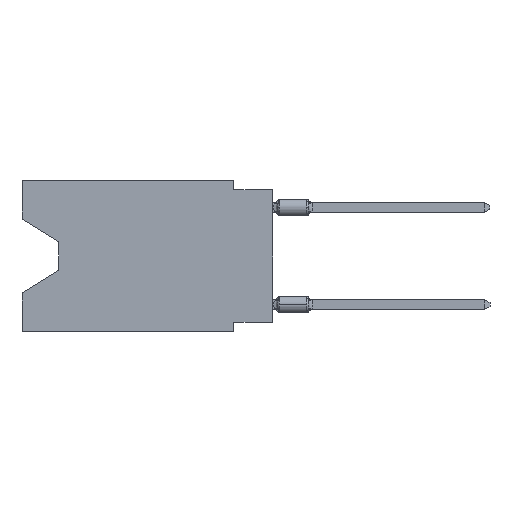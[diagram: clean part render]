
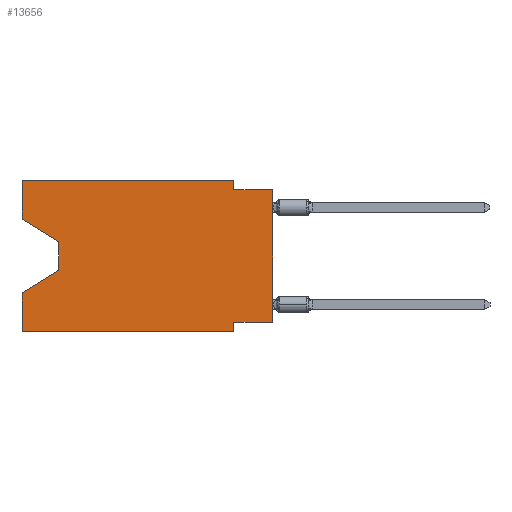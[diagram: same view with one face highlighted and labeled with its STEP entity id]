
A CAD part, left-side view. The second image highlights one B-rep face of the part: STEP entity #13656.
In plain terms, the highlighted planar face has unit normal (-1, 0, 0).
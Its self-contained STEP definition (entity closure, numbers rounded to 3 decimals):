
#213 = ORIENTED_EDGE ( 'NONE', *, *, #5521, .F. ) ;
#245 = PLANE ( 'NONE',  #2323 ) ;
#471 = LINE ( 'NONE', #8874, #9434 ) ;
#773 = LINE ( 'NONE', #6853, #8506 ) ;
#852 = DIRECTION ( 'NONE',  ( 0., 0.855, -0.519 ) ) ;
#1445 = VECTOR ( 'NONE', #23625, 1000. ) ;
#1510 = CARTESIAN_POINT ( 'NONE',  ( 0., 2.54, -9.906 ) ) ;
#1576 = CARTESIAN_POINT ( 'NONE',  ( 0., 16.383, -9.906 ) ) ;
#1768 = VECTOR ( 'NONE', #10287, 1000. ) ;
#1894 = ORIENTED_EDGE ( 'NONE', *, *, #12144, .F. ) ;
#1935 = ORIENTED_EDGE ( 'NONE', *, *, #8682, .F. ) ;
#1942 = VERTEX_POINT ( 'NONE', #14282 ) ;
#2323 = AXIS2_PLACEMENT_3D ( 'NONE', #23808, #4020, #10089 ) ;
#2403 = LINE ( 'NONE', #18314, #1768 ) ;
#2488 = CARTESIAN_POINT ( 'NONE',  ( 0., 16.383, 0. ) ) ;
#2506 = LINE ( 'NONE', #6135, #14990 ) ;
#2521 = EDGE_CURVE ( 'NONE', #8930, #2765, #773, .T. ) ;
#2765 = VERTEX_POINT ( 'NONE', #9418 ) ;
#2784 = ORIENTED_EDGE ( 'NONE', *, *, #15874, .T. ) ;
#3424 = CARTESIAN_POINT ( 'NONE',  ( 0., 2.54, 0. ) ) ;
#4020 = DIRECTION ( 'NONE',  ( 1., 0., 0. ) ) ;
#4273 = EDGE_CURVE ( 'NONE', #7052, #2765, #4348, .T. ) ;
#4348 = LINE ( 'NONE', #24664, #4438 ) ;
#4438 = VECTOR ( 'NONE', #852, 1000. ) ;
#4528 = DIRECTION ( 'NONE',  ( 0., 0., 1. ) ) ;
#5235 = LINE ( 'NONE', #3424, #25287 ) ;
#5400 = VECTOR ( 'NONE', #9411, 1000. ) ;
#5521 = EDGE_CURVE ( 'NONE', #1942, #22151, #471, .T. ) ;
#6133 = VERTEX_POINT ( 'NONE', #22689 ) ;
#6135 = CARTESIAN_POINT ( 'NONE',  ( 0., 0., -0.635 ) ) ;
#6368 = DIRECTION ( 'NONE',  ( 0., -1., 0. ) ) ;
#6853 = CARTESIAN_POINT ( 'NONE',  ( 0., 16.383, 0. ) ) ;
#7016 = EDGE_CURVE ( 'NONE', #22151, #11858, #15379, .T. ) ;
#7052 = VERTEX_POINT ( 'NONE', #24275 ) ;
#7441 = ORIENTED_EDGE ( 'NONE', *, *, #11466, .T. ) ;
#7478 = CARTESIAN_POINT ( 'NONE',  ( 0., 2.54, 0. ) ) ;
#7889 = VECTOR ( 'NONE', #24827, 1000. ) ;
#8082 = EDGE_LOOP ( 'NONE', ( #16362, #10156, #13849, #12026, #7441, #9031, #213, #2784, #1935, #17126, #1894, #15111 ) ) ;
#8506 = VECTOR ( 'NONE', #4528, 1000. ) ;
#8641 = CARTESIAN_POINT ( 'NONE',  ( 0., 13.97, -4.013 ) ) ;
#8682 = EDGE_CURVE ( 'NONE', #14234, #11019, #2506, .T. ) ;
#8874 = CARTESIAN_POINT ( 'NONE',  ( 0., 0., -9.271 ) ) ;
#8930 = VERTEX_POINT ( 'NONE', #1576 ) ;
#9031 = ORIENTED_EDGE ( 'NONE', *, *, #7016, .F. ) ;
#9411 = DIRECTION ( 'NONE',  ( 0., 0., -1. ) ) ;
#9418 = CARTESIAN_POINT ( 'NONE',  ( 0., 16.383, -7.36 ) ) ;
#9434 = VECTOR ( 'NONE', #16774, 1000. ) ;
#9471 = VERTEX_POINT ( 'NONE', #7478 ) ;
#10089 = DIRECTION ( 'NONE',  ( 0., 0., -1. ) ) ;
#10156 = ORIENTED_EDGE ( 'NONE', *, *, #19746, .T. ) ;
#10287 = DIRECTION ( 'NONE',  ( 0., 0., 1. ) ) ;
#11019 = VERTEX_POINT ( 'NONE', #18893 ) ;
#11466 = EDGE_CURVE ( 'NONE', #8930, #11858, #18868, .T. ) ;
#11720 = CARTESIAN_POINT ( 'NONE',  ( 0., 16.383, -2.546 ) ) ;
#11858 = VERTEX_POINT ( 'NONE', #25146 ) ;
#12026 = ORIENTED_EDGE ( 'NONE', *, *, #2521, .F. ) ;
#12144 = EDGE_CURVE ( 'NONE', #22793, #9471, #24092, .T. ) ;
#12272 = LINE ( 'NONE', #8641, #23276 ) ;
#13274 = CARTESIAN_POINT ( 'NONE',  ( 0., 16.383, 0. ) ) ;
#13582 = DIRECTION ( 'NONE',  ( 0., 0., 1. ) ) ;
#13656 = ADVANCED_FACE ( 'NONE', ( #23679 ), #245, .F. ) ;
#13849 = ORIENTED_EDGE ( 'NONE', *, *, #4273, .T. ) ;
#14234 = VERTEX_POINT ( 'NONE', #24159 ) ;
#14282 = CARTESIAN_POINT ( 'NONE',  ( 0., 0., -9.271 ) ) ;
#14763 = CARTESIAN_POINT ( 'NONE',  ( 0., 2.54, -9.271 ) ) ;
#14990 = VECTOR ( 'NONE', #23729, 1000. ) ;
#15111 = ORIENTED_EDGE ( 'NONE', *, *, #18962, .F. ) ;
#15379 = LINE ( 'NONE', #1510, #5400 ) ;
#15874 = EDGE_CURVE ( 'NONE', #1942, #11019, #17200, .T. ) ;
#16362 = ORIENTED_EDGE ( 'NONE', *, *, #16398, .T. ) ;
#16398 = EDGE_CURVE ( 'NONE', #6133, #21118, #21547, .T. ) ;
#16774 = DIRECTION ( 'NONE',  ( 0., 1., 0. ) ) ;
#16942 = CARTESIAN_POINT ( 'NONE',  ( 0., 16.383, -9.906 ) ) ;
#17126 = ORIENTED_EDGE ( 'NONE', *, *, #17768, .F. ) ;
#17200 = LINE ( 'NONE', #23392, #18786 ) ;
#17768 = EDGE_CURVE ( 'NONE', #9471, #14234, #5235, .T. ) ;
#18314 = CARTESIAN_POINT ( 'NONE',  ( 0., 16.383, 0. ) ) ;
#18786 = VECTOR ( 'NONE', #13582, 1000. ) ;
#18868 = LINE ( 'NONE', #16942, #7889 ) ;
#18893 = CARTESIAN_POINT ( 'NONE',  ( 0., 0., -0.635 ) ) ;
#18962 = EDGE_CURVE ( 'NONE', #6133, #22793, #2403, .T. ) ;
#19746 = EDGE_CURVE ( 'NONE', #21118, #7052, #12272, .T. ) ;
#20158 = DIRECTION ( 'NONE',  ( 0., 0., -1. ) ) ;
#21118 = VERTEX_POINT ( 'NONE', #22256 ) ;
#21547 = LINE ( 'NONE', #11720, #1445 ) ;
#22151 = VERTEX_POINT ( 'NONE', #14763 ) ;
#22256 = CARTESIAN_POINT ( 'NONE',  ( 0., 13.97, -4.013 ) ) ;
#22689 = CARTESIAN_POINT ( 'NONE',  ( 0., 16.383, -2.546 ) ) ;
#22793 = VERTEX_POINT ( 'NONE', #13274 ) ;
#23276 = VECTOR ( 'NONE', #20158, 1000. ) ;
#23392 = CARTESIAN_POINT ( 'NONE',  ( 0., 0., 0. ) ) ;
#23625 = DIRECTION ( 'NONE',  ( 0., -0.855, -0.519 ) ) ;
#23679 = FACE_OUTER_BOUND ( 'NONE', #8082, .T. ) ;
#23729 = DIRECTION ( 'NONE',  ( 0., -1., 0. ) ) ;
#23808 = CARTESIAN_POINT ( 'NONE',  ( 0., 16.383, 0. ) ) ;
#24092 = LINE ( 'NONE', #2488, #25278 ) ;
#24159 = CARTESIAN_POINT ( 'NONE',  ( 0., 2.54, -0.635 ) ) ;
#24275 = CARTESIAN_POINT ( 'NONE',  ( 0., 13.97, -5.893 ) ) ;
#24664 = CARTESIAN_POINT ( 'NONE',  ( 0., 13.97, -5.893 ) ) ;
#24779 = DIRECTION ( 'NONE',  ( 0., 0., -1. ) ) ;
#24827 = DIRECTION ( 'NONE',  ( 0., -1., 0. ) ) ;
#25146 = CARTESIAN_POINT ( 'NONE',  ( 0., 2.54, -9.906 ) ) ;
#25278 = VECTOR ( 'NONE', #6368, 1000. ) ;
#25287 = VECTOR ( 'NONE', #24779, 1000. ) ;
